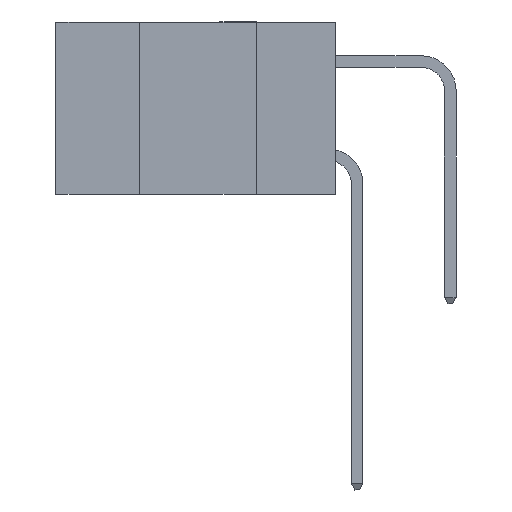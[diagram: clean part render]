
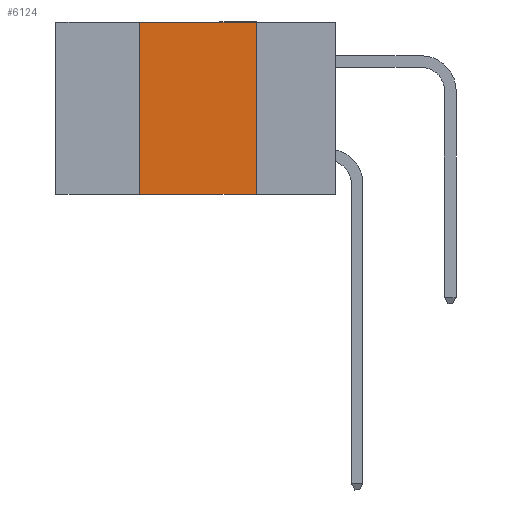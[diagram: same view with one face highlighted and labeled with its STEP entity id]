
A CAD part, left-side view. The second image highlights one B-rep face of the part: STEP entity #6124.
In plain terms, the highlighted planar face has unit normal (-1, 0, 0).
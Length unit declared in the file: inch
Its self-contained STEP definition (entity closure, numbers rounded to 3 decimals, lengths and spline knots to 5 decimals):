
#156 = CARTESIAN_POINT ( 'NONE',  ( 0., 0.17, 0. ) ) ;
#546 = CARTESIAN_POINT ( 'NONE',  ( 0., 0.42, 0. ) ) ;
#753 = ORIENTED_EDGE ( 'NONE', *, *, #8099, .T. ) ;
#901 = LINE ( 'NONE', #156, #3639 ) ;
#1237 = CARTESIAN_POINT ( 'NONE',  ( 0., 0.42, -0.37 ) ) ;
#1677 = PLANE ( 'NONE',  #8165 ) ;
#1724 = EDGE_CURVE ( 'NONE', #3536, #6009, #3660, .T. ) ;
#1953 = VECTOR ( 'NONE', #3952, 39.37008 ) ;
#2481 = EDGE_LOOP ( 'NONE', ( #10402, #5644, #4514, #753 ) ) ;
#2537 = DIRECTION ( 'NONE',  ( 1., 0., 0. ) ) ;
#2969 = CARTESIAN_POINT ( 'NONE',  ( 0., 0.6, -0.37 ) ) ;
#3090 = DIRECTION ( 'NONE',  ( 0., -1., 0. ) ) ;
#3451 = FACE_OUTER_BOUND ( 'NONE', #2481, .T. ) ;
#3536 = VERTEX_POINT ( 'NONE', #546 ) ;
#3639 = VECTOR ( 'NONE', #5143, 39.37008 ) ;
#3660 = LINE ( 'NONE', #8946, #1953 ) ;
#3952 = DIRECTION ( 'NONE',  ( 0., -1., 0. ) ) ;
#4514 = ORIENTED_EDGE ( 'NONE', *, *, #8692, .F. ) ;
#5065 = LINE ( 'NONE', #6274, #8285 ) ;
#5143 = DIRECTION ( 'NONE',  ( 0., 0., -1. ) ) ;
#5644 = ORIENTED_EDGE ( 'NONE', *, *, #1724, .F. ) ;
#5979 = CARTESIAN_POINT ( 'NONE',  ( 0., 0.17, -0.37 ) ) ;
#6009 = VERTEX_POINT ( 'NONE', #9750 ) ;
#6124 = ADVANCED_FACE ( 'NONE', ( #3451 ), #1677, .F. ) ;
#6137 = DIRECTION ( 'NONE',  ( 0., 0., 1. ) ) ;
#6274 = CARTESIAN_POINT ( 'NONE',  ( 0., 0.42, 0. ) ) ;
#6500 = VECTOR ( 'NONE', #3090, 39.37008 ) ;
#6766 = CARTESIAN_POINT ( 'NONE',  ( 0., 0.6, 0. ) ) ;
#7602 = DIRECTION ( 'NONE',  ( 0., 0., -1. ) ) ;
#8099 = EDGE_CURVE ( 'NONE', #8644, #9102, #9873, .T. ) ;
#8165 = AXIS2_PLACEMENT_3D ( 'NONE', #6766, #2537, #7602 ) ;
#8285 = VECTOR ( 'NONE', #6137, 39.37008 ) ;
#8644 = VERTEX_POINT ( 'NONE', #1237 ) ;
#8692 = EDGE_CURVE ( 'NONE', #8644, #3536, #5065, .T. ) ;
#8946 = CARTESIAN_POINT ( 'NONE',  ( 0., 0.6, 0. ) ) ;
#9066 = EDGE_CURVE ( 'NONE', #6009, #9102, #901, .T. ) ;
#9102 = VERTEX_POINT ( 'NONE', #5979 ) ;
#9750 = CARTESIAN_POINT ( 'NONE',  ( 0., 0.17, 0. ) ) ;
#9873 = LINE ( 'NONE', #2969, #6500 ) ;
#10402 = ORIENTED_EDGE ( 'NONE', *, *, #9066, .F. ) ;
